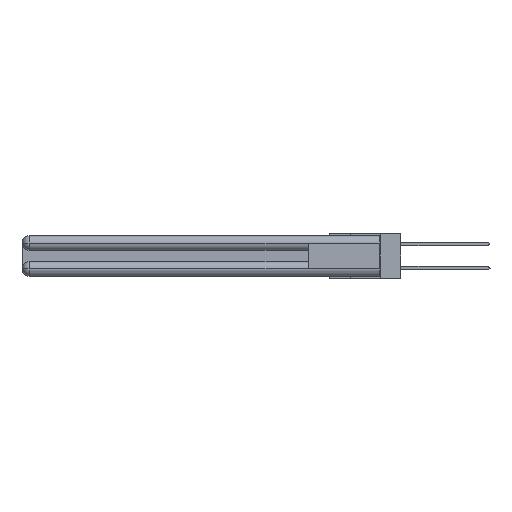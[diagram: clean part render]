
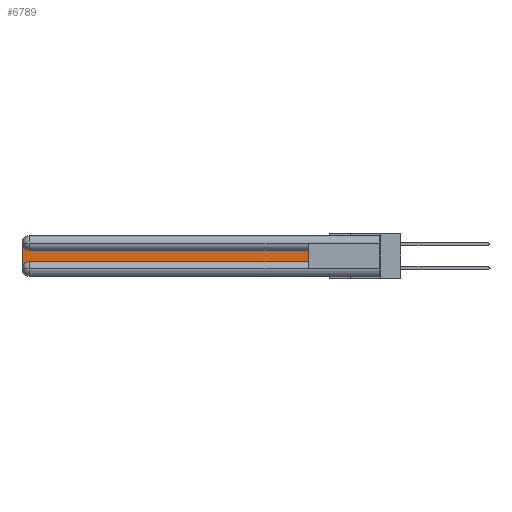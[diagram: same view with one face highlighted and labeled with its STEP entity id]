
A CAD part, left-side view. The second image highlights one B-rep face of the part: STEP entity #6789.
In plain terms, the highlighted planar face has unit normal (-1, 0, 0).
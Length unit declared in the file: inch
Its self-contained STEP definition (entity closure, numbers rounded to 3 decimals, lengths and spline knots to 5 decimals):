
#2116 = CARTESIAN_POINT ( 'NONE',  ( 0.075, 3., -0.0625 ) ) ;
#2977 = EDGE_CURVE ( 'NONE', #33145, #9983, #12205, .T. ) ;
#3749 = AXIS2_PLACEMENT_3D ( 'NONE', #29534, #5416, #18985 ) ;
#4708 = VERTEX_POINT ( 'NONE', #2116 ) ;
#4834 = CARTESIAN_POINT ( 'NONE',  ( 0.075, 2.94, -0.1225 ) ) ;
#5416 = DIRECTION ( 'NONE',  ( 1., 0., 0. ) ) ;
#6641 = CARTESIAN_POINT ( 'NONE',  ( 0.075, 3., -0.2775 ) ) ;
#6714 = EDGE_CURVE ( 'NONE', #27410, #31798, #12890, .T. ) ;
#6789 = ADVANCED_FACE ( 'NONE', ( #21817 ), #21098, .F. ) ;
#7078 = EDGE_CURVE ( 'NONE', #15240, #4708, #21784, .T. ) ;
#7620 = LINE ( 'NONE', #22903, #31437 ) ;
#8455 = ORIENTED_EDGE ( 'NONE', *, *, #7078, .T. ) ;
#9711 = LINE ( 'NONE', #27566, #18673 ) ;
#9983 = VERTEX_POINT ( 'NONE', #33265 ) ;
#10279 = DIRECTION ( 'NONE',  ( 0., 0., -1. ) ) ;
#10311 = DIRECTION ( 'NONE',  ( 0., 1., 0. ) ) ;
#12205 = LINE ( 'NONE', #27791, #30441 ) ;
#12557 = DIRECTION ( 'NONE',  ( 0., 0., -1. ) ) ;
#12890 = CIRCLE ( 'NONE', #13544, 0.06 ) ;
#12990 = ORIENTED_EDGE ( 'NONE', *, *, #23977, .T. ) ;
#13544 = AXIS2_PLACEMENT_3D ( 'NONE', #20751, #20982, #12557 ) ;
#15174 = ORIENTED_EDGE ( 'NONE', *, *, #2977, .T. ) ;
#15240 = VERTEX_POINT ( 'NONE', #4834 ) ;
#16429 = CARTESIAN_POINT ( 'NONE',  ( 0.075, 2.94, -0.2175 ) ) ;
#16434 = LINE ( 'NONE', #26586, #17296 ) ;
#16595 = CARTESIAN_POINT ( 'NONE',  ( 0.075, 0.6, -0.2175 ) ) ;
#17296 = VECTOR ( 'NONE', #10311, 39.37008 ) ;
#18132 = CARTESIAN_POINT ( 'NONE',  ( 0.075, 3., -0.1225 ) ) ;
#18673 = VECTOR ( 'NONE', #21292, 39.37008 ) ;
#18773 = EDGE_LOOP ( 'NONE', ( #34888, #8455, #12990, #31295, #31112, #15174 ) ) ;
#18985 = DIRECTION ( 'NONE',  ( 0., 0., -1. ) ) ;
#19657 = EDGE_CURVE ( 'NONE', #9983, #15240, #16434, .T. ) ;
#20751 = CARTESIAN_POINT ( 'NONE',  ( 0.075, 2.94, -0.2775 ) ) ;
#20982 = DIRECTION ( 'NONE',  ( 1., 0., 0. ) ) ;
#21098 = PLANE ( 'NONE',  #30380 ) ;
#21292 = DIRECTION ( 'NONE',  ( 0., -1., 0. ) ) ;
#21784 = CIRCLE ( 'NONE', #3749, 0.06 ) ;
#21817 = FACE_OUTER_BOUND ( 'NONE', #18773, .T. ) ;
#22903 = CARTESIAN_POINT ( 'NONE',  ( 0.075, 3., -0.2175 ) ) ;
#23977 = EDGE_CURVE ( 'NONE', #4708, #27410, #7620, .T. ) ;
#24495 = EDGE_CURVE ( 'NONE', #31798, #33145, #9711, .T. ) ;
#26586 = CARTESIAN_POINT ( 'NONE',  ( 0.075, 0.6, -0.1225 ) ) ;
#27410 = VERTEX_POINT ( 'NONE', #6641 ) ;
#27566 = CARTESIAN_POINT ( 'NONE',  ( 0.075, 0.6, -0.2175 ) ) ;
#27791 = CARTESIAN_POINT ( 'NONE',  ( 0.075, 0.6, -0.2175 ) ) ;
#27905 = DIRECTION ( 'NONE',  ( 0., 0., 1. ) ) ;
#29534 = CARTESIAN_POINT ( 'NONE',  ( 0.075, 2.94, -0.0625 ) ) ;
#30380 = AXIS2_PLACEMENT_3D ( 'NONE', #18132, #31784, #10279 ) ;
#30441 = VECTOR ( 'NONE', #27905, 39.37008 ) ;
#31112 = ORIENTED_EDGE ( 'NONE', *, *, #24495, .T. ) ;
#31295 = ORIENTED_EDGE ( 'NONE', *, *, #6714, .T. ) ;
#31437 = VECTOR ( 'NONE', #33604, 39.37008 ) ;
#31784 = DIRECTION ( 'NONE',  ( 1., 0., 0. ) ) ;
#31798 = VERTEX_POINT ( 'NONE', #16429 ) ;
#33145 = VERTEX_POINT ( 'NONE', #16595 ) ;
#33265 = CARTESIAN_POINT ( 'NONE',  ( 0.075, 0.6, -0.1225 ) ) ;
#33604 = DIRECTION ( 'NONE',  ( 0., 0., -1. ) ) ;
#34888 = ORIENTED_EDGE ( 'NONE', *, *, #19657, .T. ) ;
